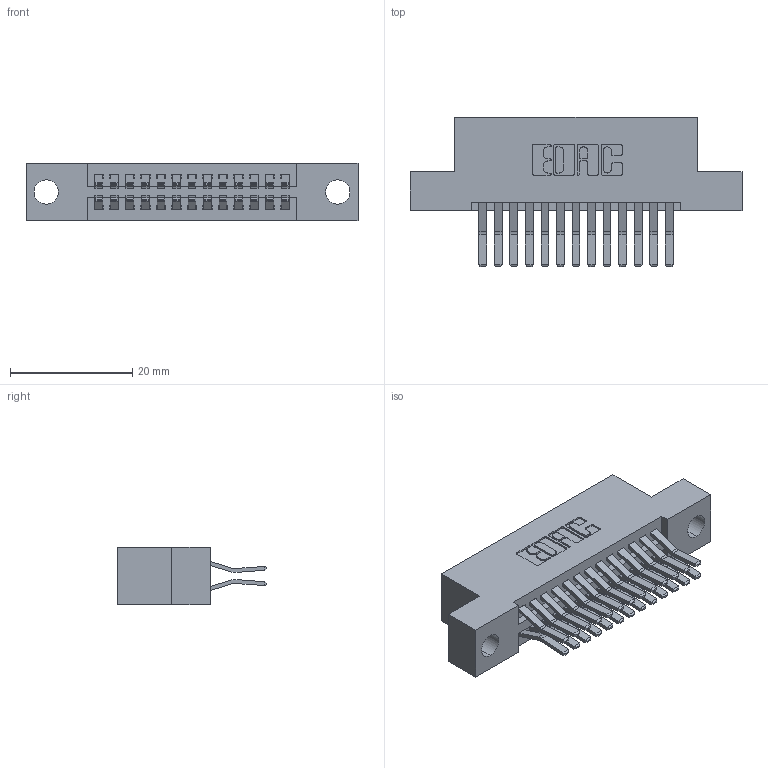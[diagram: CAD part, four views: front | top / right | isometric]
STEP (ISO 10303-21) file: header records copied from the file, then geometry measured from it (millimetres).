
FILE_DESCRIPTION (( 'STEP AP203' ), '1' );
FILE_NAME ('395-026-560-204.STEP', '2021-06-16T19:39:52', ( '' ), ( '' ), 'SwSTEP 2.0', 'SolidWorks 2020', '' );
FILE_SCHEMA (( 'CONFIG_CONTROL_DESIGN' ));
Length unit declared in the file: inch
Products named in the file (3): 395-026-560-204; 345-292-001_560 Tail; 345 Part_Flush Mounting Lugs - 0.156 Dia-TI
Assembly tree (27 placements, depth 2):
  395-026-560-204
    345 Part_Flush Mounting Lugs - 0.156 Dia-TI
    345-292-001_560 Tail  x26
Bounding box: 54.23 x 24.45 x 9.4 mm (x, y, z)
Volume: 5063.1 mm3; surface area: 7212.4 mm2
Topology: 27 solids, 27 shells, 1492 faces, 4407 edges, 2902 vertices
Faces by surface type: plane 952, cylinder 540
Entity records: 14611 total; most frequent: CARTESIAN_POINT 2482, ORIENTED_EDGE 2414, DIRECTION 2227, EDGE_CURVE 1207, VECTOR 1019, LINE 1019, VERTEX_POINT 802, AXIS2_PLACEMENT_3D 604
